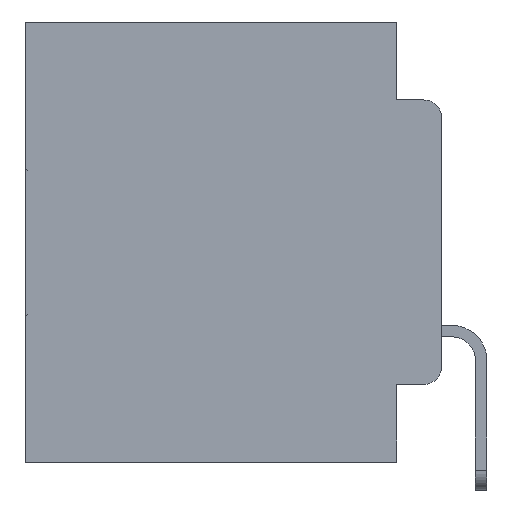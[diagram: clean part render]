
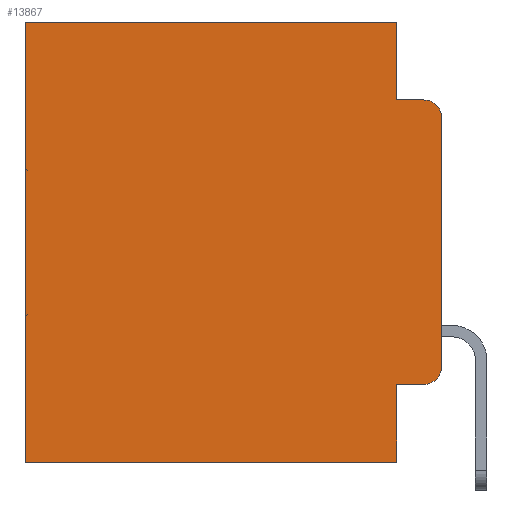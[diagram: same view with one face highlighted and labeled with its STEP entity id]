
A CAD part, left-side view. The second image highlights one B-rep face of the part: STEP entity #13867.
In plain terms, the highlighted planar face has unit normal (-1, 0, 0).
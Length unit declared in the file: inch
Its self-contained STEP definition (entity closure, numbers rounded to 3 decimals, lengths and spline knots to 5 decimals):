
#270 = ORIENTED_EDGE ( 'NONE', *, *, #27502, .F. ) ;
#319 = ORIENTED_EDGE ( 'NONE', *, *, #14850, .T. ) ;
#479 = EDGE_CURVE ( 'NONE', #8678, #10957, #27038, .T. ) ;
#607 = DIRECTION ( 'NONE',  ( 0., -1., 0. ) ) ;
#811 = DIRECTION ( 'NONE',  ( 0., 0., -1. ) ) ;
#814 = CARTESIAN_POINT ( 'NONE',  ( 0.298, 0.02, -0.3915 ) ) ;
#1369 = CARTESIAN_POINT ( 'NONE',  ( 0.298, 0.473, -0.5 ) ) ;
#2046 = VERTEX_POINT ( 'NONE', #6270 ) ;
#2171 = VERTEX_POINT ( 'NONE', #27717 ) ;
#2421 = VERTEX_POINT ( 'NONE', #5701 ) ;
#2453 = VERTEX_POINT ( 'NONE', #24732 ) ;
#2823 = EDGE_CURVE ( 'NONE', #6412, #2421, #27896, .T. ) ;
#2837 = DIRECTION ( 'NONE',  ( 0., 1., 0. ) ) ;
#3175 = VERTEX_POINT ( 'NONE', #4849 ) ;
#3406 = DIRECTION ( 'NONE',  ( 0., 0., -1. ) ) ;
#3480 = LINE ( 'NONE', #5394, #15827 ) ;
#3755 = CIRCLE ( 'NONE', #10490, 0.02 ) ;
#4849 = CARTESIAN_POINT ( 'NONE',  ( 0.298, 0., -0.1085 ) ) ;
#5394 = CARTESIAN_POINT ( 'NONE',  ( 0.298, 0., -0.5 ) ) ;
#5701 = CARTESIAN_POINT ( 'NONE',  ( 0.298, 0.051, -0.5 ) ) ;
#5857 = EDGE_CURVE ( 'NONE', #3175, #2171, #19874, .T. ) ;
#5986 = AXIS2_PLACEMENT_3D ( 'NONE', #814, #18018, #3406 ) ;
#5993 = DIRECTION ( 'NONE',  ( 0., 0., -1. ) ) ;
#6075 = ORIENTED_EDGE ( 'NONE', *, *, #11152, .T. ) ;
#6208 = DIRECTION ( 'NONE',  ( 0., 1., 0. ) ) ;
#6270 = CARTESIAN_POINT ( 'NONE',  ( 0.298, 0.473, 0. ) ) ;
#6397 = FACE_OUTER_BOUND ( 'NONE', #24720, .T. ) ;
#6412 = VERTEX_POINT ( 'NONE', #22849 ) ;
#6765 = ORIENTED_EDGE ( 'NONE', *, *, #8469, .T. ) ;
#7189 = LINE ( 'NONE', #13043, #19235 ) ;
#7749 = AXIS2_PLACEMENT_3D ( 'NONE', #29082, #15690, #811 ) ;
#8272 = PLANE ( 'NONE',  #7749 ) ;
#8469 = EDGE_CURVE ( 'NONE', #2453, #2171, #16158, .T. ) ;
#8678 = VERTEX_POINT ( 'NONE', #25611 ) ;
#9510 = VECTOR ( 'NONE', #28926, 39.37008 ) ;
#10382 = EDGE_CURVE ( 'NONE', #2421, #13429, #3480, .T. ) ;
#10490 = AXIS2_PLACEMENT_3D ( 'NONE', #11549, #27580, #14049 ) ;
#10599 = DIRECTION ( 'NONE',  ( 0., -1., 0. ) ) ;
#10957 = VERTEX_POINT ( 'NONE', #29051 ) ;
#11152 = EDGE_CURVE ( 'NONE', #2046, #13429, #24921, .T. ) ;
#11549 = CARTESIAN_POINT ( 'NONE',  ( 0.298, 0.02, -0.1085 ) ) ;
#13043 = CARTESIAN_POINT ( 'NONE',  ( 0.298, 0.051, -0.4115 ) ) ;
#13429 = VERTEX_POINT ( 'NONE', #1369 ) ;
#13867 = ADVANCED_FACE ( 'NONE', ( #6397 ), #8272, .F. ) ;
#14049 = DIRECTION ( 'NONE',  ( 0., 0., -1. ) ) ;
#14850 = EDGE_CURVE ( 'NONE', #8678, #2046, #19473, .T. ) ;
#15297 = ORIENTED_EDGE ( 'NONE', *, *, #2823, .F. ) ;
#15690 = DIRECTION ( 'NONE',  ( 1., 0., 0. ) ) ;
#15827 = VECTOR ( 'NONE', #2837, 39.37008 ) ;
#16158 = CIRCLE ( 'NONE', #5986, 0.02 ) ;
#16291 = ORIENTED_EDGE ( 'NONE', *, *, #10382, .F. ) ;
#17967 = VERTEX_POINT ( 'NONE', #29325 ) ;
#18018 = DIRECTION ( 'NONE',  ( -1., 0., 0. ) ) ;
#19235 = VECTOR ( 'NONE', #607, 39.37008 ) ;
#19250 = ORIENTED_EDGE ( 'NONE', *, *, #27866, .T. ) ;
#19473 = LINE ( 'NONE', #25005, #30564 ) ;
#19874 = LINE ( 'NONE', #26916, #25135 ) ;
#21632 = ORIENTED_EDGE ( 'NONE', *, *, #479, .F. ) ;
#21661 = ORIENTED_EDGE ( 'NONE', *, *, #24168, .T. ) ;
#22275 = CARTESIAN_POINT ( 'NONE',  ( 0.298, 0.051, 0. ) ) ;
#22849 = CARTESIAN_POINT ( 'NONE',  ( 0.298, 0.051, -0.4115 ) ) ;
#23164 = LINE ( 'NONE', #26721, #23853 ) ;
#23268 = DIRECTION ( 'NONE',  ( 0., 0., -1. ) ) ;
#23853 = VECTOR ( 'NONE', #10599, 39.37008 ) ;
#24168 = EDGE_CURVE ( 'NONE', #6412, #2453, #7189, .T. ) ;
#24210 = VECTOR ( 'NONE', #23268, 39.37008 ) ;
#24720 = EDGE_LOOP ( 'NONE', ( #26414, #19250, #270, #21632, #319, #6075, #16291, #15297, #21661, #6765 ) ) ;
#24732 = CARTESIAN_POINT ( 'NONE',  ( 0.298, 0.02, -0.4115 ) ) ;
#24921 = LINE ( 'NONE', #25479, #24210 ) ;
#25005 = CARTESIAN_POINT ( 'NONE',  ( 0.298, 0., 0. ) ) ;
#25135 = VECTOR ( 'NONE', #5993, 39.37008 ) ;
#25479 = CARTESIAN_POINT ( 'NONE',  ( 0.298, 0.473, 0. ) ) ;
#25611 = CARTESIAN_POINT ( 'NONE',  ( 0.298, 0.051, 0. ) ) ;
#26330 = VECTOR ( 'NONE', #28129, 39.37008 ) ;
#26414 = ORIENTED_EDGE ( 'NONE', *, *, #5857, .F. ) ;
#26721 = CARTESIAN_POINT ( 'NONE',  ( 0.298, 0.051, -0.0885 ) ) ;
#26916 = CARTESIAN_POINT ( 'NONE',  ( 0.298, 0., 0. ) ) ;
#27038 = LINE ( 'NONE', #27080, #26330 ) ;
#27080 = CARTESIAN_POINT ( 'NONE',  ( 0.298, 0.051, 0. ) ) ;
#27502 = EDGE_CURVE ( 'NONE', #10957, #17967, #23164, .T. ) ;
#27580 = DIRECTION ( 'NONE',  ( -1., 0., 0. ) ) ;
#27717 = CARTESIAN_POINT ( 'NONE',  ( 0.298, 0., -0.3915 ) ) ;
#27866 = EDGE_CURVE ( 'NONE', #3175, #17967, #3755, .T. ) ;
#27896 = LINE ( 'NONE', #22275, #9510 ) ;
#28129 = DIRECTION ( 'NONE',  ( 0., 0., -1. ) ) ;
#28926 = DIRECTION ( 'NONE',  ( 0., 0., -1. ) ) ;
#29051 = CARTESIAN_POINT ( 'NONE',  ( 0.298, 0.051, -0.0885 ) ) ;
#29082 = CARTESIAN_POINT ( 'NONE',  ( 0.298, 0., 0. ) ) ;
#29325 = CARTESIAN_POINT ( 'NONE',  ( 0.298, 0.02, -0.0885 ) ) ;
#30564 = VECTOR ( 'NONE', #6208, 39.37008 ) ;
